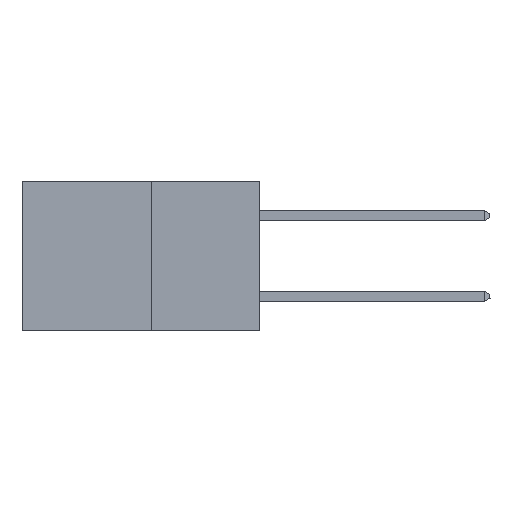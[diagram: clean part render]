
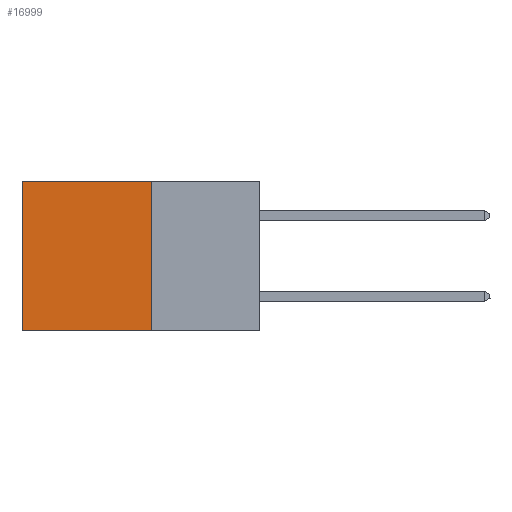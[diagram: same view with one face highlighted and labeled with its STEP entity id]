
A CAD part, left-side view. The second image highlights one B-rep face of the part: STEP entity #16999.
In plain terms, the highlighted planar face has unit normal (-1, 0, 0).
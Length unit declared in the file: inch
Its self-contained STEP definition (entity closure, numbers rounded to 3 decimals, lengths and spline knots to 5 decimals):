
#584 = LINE ( 'NONE', #6977, #25135 ) ;
#3341 = ORIENTED_EDGE ( 'NONE', *, *, #25870, .F. ) ;
#3469 = VERTEX_POINT ( 'NONE', #13264 ) ;
#4920 = DIRECTION ( 'NONE',  ( 0., 0., -1. ) ) ;
#5138 = EDGE_CURVE ( 'NONE', #17527, #21225, #584, .T. ) ;
#5320 = DIRECTION ( 'NONE',  ( 0., 1., 0. ) ) ;
#5701 = CARTESIAN_POINT ( 'NONE',  ( 0.277, 0.27, -0.37 ) ) ;
#6123 = ORIENTED_EDGE ( 'NONE', *, *, #5138, .T. ) ;
#6219 = CARTESIAN_POINT ( 'NONE',  ( 0.277, 0.27, -0.37 ) ) ;
#6825 = EDGE_CURVE ( 'NONE', #21225, #3469, #15869, .T. ) ;
#6977 = CARTESIAN_POINT ( 'NONE',  ( 0.277, 0.27, 0. ) ) ;
#7121 = LINE ( 'NONE', #19144, #13466 ) ;
#8115 = PLANE ( 'NONE',  #14273 ) ;
#9580 = VECTOR ( 'NONE', #18054, 39.37008 ) ;
#10422 = ORIENTED_EDGE ( 'NONE', *, *, #6825, .T. ) ;
#10506 = DIRECTION ( 'NONE',  ( 1., 0., 0. ) ) ;
#13264 = CARTESIAN_POINT ( 'NONE',  ( 0.277, 0.59, -0.37 ) ) ;
#13346 = VERTEX_POINT ( 'NONE', #6219 ) ;
#13378 = LINE ( 'NONE', #28068, #18126 ) ;
#13466 = VECTOR ( 'NONE', #4920, 39.37008 ) ;
#14273 = AXIS2_PLACEMENT_3D ( 'NONE', #5701, #10506, #26966 ) ;
#14830 = FACE_OUTER_BOUND ( 'NONE', #21504, .T. ) ;
#15869 = LINE ( 'NONE', #18416, #9580 ) ;
#16999 = ADVANCED_FACE ( 'NONE', ( #14830 ), #8115, .F. ) ;
#17527 = VERTEX_POINT ( 'NONE', #26427 ) ;
#18054 = DIRECTION ( 'NONE',  ( 0., 0., -1. ) ) ;
#18126 = VECTOR ( 'NONE', #30415, 39.37008 ) ;
#18416 = CARTESIAN_POINT ( 'NONE',  ( 0.277, 0.59, -0.37 ) ) ;
#19144 = CARTESIAN_POINT ( 'NONE',  ( 0.277, 0.27, -0.37 ) ) ;
#21225 = VERTEX_POINT ( 'NONE', #30530 ) ;
#21504 = EDGE_LOOP ( 'NONE', ( #10422, #26224, #3341, #6123 ) ) ;
#25135 = VECTOR ( 'NONE', #5320, 39.37008 ) ;
#25870 = EDGE_CURVE ( 'NONE', #17527, #13346, #7121, .T. ) ;
#26224 = ORIENTED_EDGE ( 'NONE', *, *, #28622, .F. ) ;
#26427 = CARTESIAN_POINT ( 'NONE',  ( 0.277, 0.27, 0. ) ) ;
#26966 = DIRECTION ( 'NONE',  ( 0., 0., -1. ) ) ;
#28068 = CARTESIAN_POINT ( 'NONE',  ( 0.277, 0.27, -0.37 ) ) ;
#28622 = EDGE_CURVE ( 'NONE', #13346, #3469, #13378, .T. ) ;
#30415 = DIRECTION ( 'NONE',  ( 0., 1., 0. ) ) ;
#30530 = CARTESIAN_POINT ( 'NONE',  ( 0.277, 0.59, 0. ) ) ;
